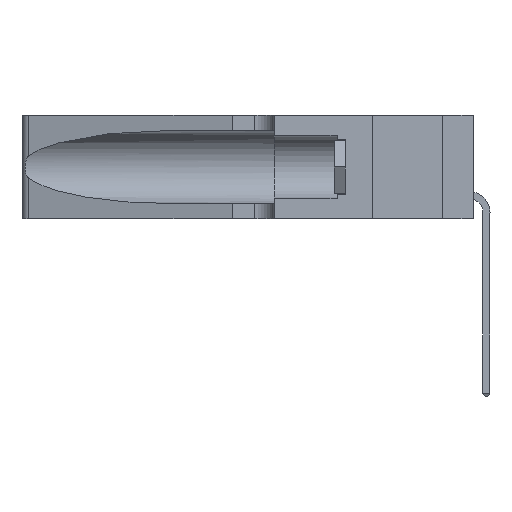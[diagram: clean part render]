
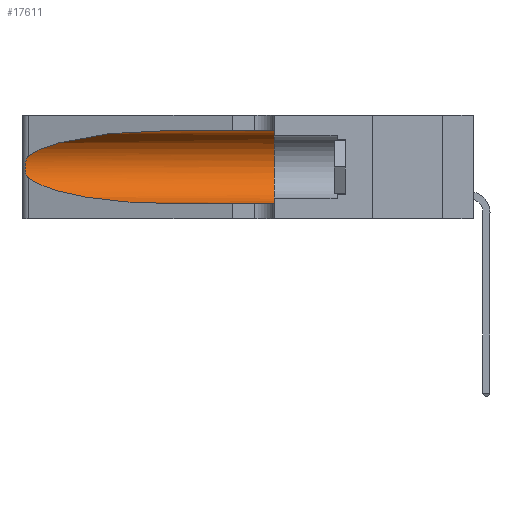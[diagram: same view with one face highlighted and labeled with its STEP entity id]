
A CAD part, left-side view. The second image highlights one B-rep face of the part: STEP entity #17611.
In plain terms, the highlighted cylindrical face has radius 3.308 mm (diameter 6.617 mm), a partial arc.
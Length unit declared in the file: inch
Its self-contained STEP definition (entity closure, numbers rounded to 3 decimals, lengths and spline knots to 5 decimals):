
#126 = VECTOR ( 'NONE', #10944, 39.37008 ) ;
#475 = CARTESIAN_POINT ( 'NONE',  ( 0.25854, 1.2359, 0.20912 ) ) ;
#480 = LINE ( 'NONE', #24969, #126 ) ;
#742 = CARTESIAN_POINT ( 'NONE',  ( 0.25487, 1.22718, 0.14631 ) ) ;
#2258 = CARTESIAN_POINT ( 'NONE',  ( 0.25487, 1.22718, 0.22369 ) ) ;
#2458 = CARTESIAN_POINT ( 'NONE',  ( 0.1305, 0.72297, 0.31525 ) ) ;
#2747 = VERTEX_POINT ( 'NONE', #2458 ) ;
#3385 = CARTESIAN_POINT ( 'NONE',  ( 0.18966, 0.96281, 0.05475 ) ) ;
#4242 = CIRCLE ( 'NONE', #4570, 0.13025 ) ;
#4348 = VERTEX_POINT ( 'NONE', #22023 ) ;
#4570 = AXIS2_PLACEMENT_3D ( 'NONE', #25938, #28212, #21533 ) ;
#4676 = CARTESIAN_POINT ( 'NONE',  ( 0.2373, 1.15595, 0.28018 ) ) ;
#5345 = CYLINDRICAL_SURFACE ( 'NONE', #11756, 0.13025 ) ;
#5872 =( BOUNDED_CURVE ( )  B_SPLINE_CURVE ( 3, ( #13758, #20912, #4676, #2258 ),
 .UNSPECIFIED., .F., .F. ) 
 B_SPLINE_CURVE_WITH_KNOTS ( ( 4, 4 ),
 ( 1.5708, 2.84003 ),
 .UNSPECIFIED. ) 
 CURVE ( )  GEOMETRIC_REPRESENTATION_ITEM ( )  RATIONAL_B_SPLINE_CURVE ( ( 1., 0.87, 0.87, 1. ) ) 
 REPRESENTATION_ITEM ( '' )  );
#6818 = CARTESIAN_POINT ( 'NONE',  ( 0.25487, 1.22718, 0.22369 ) ) ;
#7081 = CARTESIAN_POINT ( 'NONE',  ( 0.25487, 1.22718, 0.22369 ) ) ;
#7170 = CARTESIAN_POINT ( 'NONE',  ( 0.26075, 1.23896, 0.19203 ) ) ;
#7702 = LINE ( 'NONE', #16544, #13161 ) ;
#8995 = FACE_OUTER_BOUND ( 'NONE', #12289, .T. ) ;
#9411 = CARTESIAN_POINT ( 'NONE',  ( 0.25787, 1.23484, 0.2124 ) ) ;
#9726 = CARTESIAN_POINT ( 'NONE',  ( 0.25789, 1.23486, 0.15765 ) ) ;
#9734 = DIRECTION ( 'NONE',  ( 0., -1., 0. ) ) ;
#10086 = CARTESIAN_POINT ( 'NONE',  ( 0.1305, 0.72297, 0.05475 ) ) ;
#10373 = VERTEX_POINT ( 'NONE', #24013 ) ;
#10944 = DIRECTION ( 'NONE',  ( 0., -1., 0. ) ) ;
#11756 = AXIS2_PLACEMENT_3D ( 'NONE', #20277, #27458, #20471 ) ;
#11760 = CARTESIAN_POINT ( 'NONE',  ( 0.25487, 1.22718, 0.14631 ) ) ;
#11892 = ORIENTED_EDGE ( 'NONE', *, *, #30269, .F. ) ;
#12064 = CARTESIAN_POINT ( 'NONE',  ( 0.25555, 1.22993, 0.14849 ) ) ;
#12289 = EDGE_LOOP ( 'NONE', ( #15261, #12811, #27939, #25535, #11892, #27563 ) ) ;
#12811 = ORIENTED_EDGE ( 'NONE', *, *, #29656, .T. ) ;
#12876 = EDGE_CURVE ( 'NONE', #2747, #17040, #7702, .T. ) ;
#13161 = VECTOR ( 'NONE', #9734, 39.37008 ) ;
#13758 = CARTESIAN_POINT ( 'NONE',  ( 0.1305, 0.72297, 0.31525 ) ) ;
#15035 = CARTESIAN_POINT ( 'NONE',  ( 0.1305, 0.35, 0.31525 ) ) ;
#15261 = ORIENTED_EDGE ( 'NONE', *, *, #25321, .T. ) ;
#15842 = VERTEX_POINT ( 'NONE', #6818 ) ;
#16496 =( BOUNDED_CURVE ( )  B_SPLINE_CURVE ( 3, ( #742, #17305, #3385, #10086 ),
 .UNSPECIFIED., .F., .F. ) 
 B_SPLINE_CURVE_WITH_KNOTS ( ( 4, 4 ),
 ( 3.44316, 4.71239 ),
 .UNSPECIFIED. ) 
 CURVE ( )  GEOMETRIC_REPRESENTATION_ITEM ( )  RATIONAL_B_SPLINE_CURVE ( ( 1., 0.87, 0.87, 1. ) ) 
 REPRESENTATION_ITEM ( '' )  );
#16544 = CARTESIAN_POINT ( 'NONE',  ( 0.1305, 1.61858, 0.31525 ) ) ;
#17040 = VERTEX_POINT ( 'NONE', #15035 ) ;
#17305 = CARTESIAN_POINT ( 'NONE',  ( 0.2373, 1.15595, 0.08982 ) ) ;
#17611 = ADVANCED_FACE ( 'NONE', ( #8995 ), #5345, .F. ) ;
#19512 = B_SPLINE_CURVE_WITH_KNOTS ( 'NONE', 3,
 ( #7081, #25869, #28455, #9411, #475, #28153, #7170, #21375, #25780, #23752, #9726, #23541, #12064, #11760 ),
 .UNSPECIFIED., .F., .F.,
 ( 4, 2, 2, 2, 2, 2, 4 ),
 ( 0., 0.00027, 0.00053, 0.00107, 0.0016, 0.00187, 0.00214 ),
 .UNSPECIFIED. ) ;
#20108 = EDGE_CURVE ( 'NONE', #10373, #22049, #480, .T. ) ;
#20277 = CARTESIAN_POINT ( 'NONE',  ( 0.1305, 1.61858, 0.185 ) ) ;
#20471 = DIRECTION ( 'NONE',  ( 0., 0., -1. ) ) ;
#20912 = CARTESIAN_POINT ( 'NONE',  ( 0.18966, 0.96281, 0.31525 ) ) ;
#21375 = CARTESIAN_POINT ( 'NONE',  ( 0.26075, 1.23896, 0.178 ) ) ;
#21533 = DIRECTION ( 'NONE',  ( 0., 0., 1. ) ) ;
#22023 = CARTESIAN_POINT ( 'NONE',  ( 0.25487, 1.22718, 0.14631 ) ) ;
#22049 = VERTEX_POINT ( 'NONE', #22128 ) ;
#22128 = CARTESIAN_POINT ( 'NONE',  ( 0.1305, 0.35, 0.05475 ) ) ;
#23541 = CARTESIAN_POINT ( 'NONE',  ( 0.25639, 1.23186, 0.15144 ) ) ;
#23719 = EDGE_CURVE ( 'NONE', #4348, #10373, #16496, .T. ) ;
#23752 = CARTESIAN_POINT ( 'NONE',  ( 0.25856, 1.23593, 0.16098 ) ) ;
#24013 = CARTESIAN_POINT ( 'NONE',  ( 0.1305, 0.72297, 0.05475 ) ) ;
#24969 = CARTESIAN_POINT ( 'NONE',  ( 0.1305, 1.61858, 0.05475 ) ) ;
#25321 = EDGE_CURVE ( 'NONE', #2747, #15842, #5872, .T. ) ;
#25535 = ORIENTED_EDGE ( 'NONE', *, *, #20108, .T. ) ;
#25780 = CARTESIAN_POINT ( 'NONE',  ( 0.26017, 1.23833, 0.17102 ) ) ;
#25869 = CARTESIAN_POINT ( 'NONE',  ( 0.25555, 1.22994, 0.2215 ) ) ;
#25938 = CARTESIAN_POINT ( 'NONE',  ( 0.1305, 0.35, 0.185 ) ) ;
#27458 = DIRECTION ( 'NONE',  ( 0., -1., 0. ) ) ;
#27563 = ORIENTED_EDGE ( 'NONE', *, *, #12876, .F. ) ;
#27939 = ORIENTED_EDGE ( 'NONE', *, *, #23719, .T. ) ;
#28153 = CARTESIAN_POINT ( 'NONE',  ( 0.26018, 1.23835, 0.19895 ) ) ;
#28212 = DIRECTION ( 'NONE',  ( 0., 1., 0. ) ) ;
#28455 = CARTESIAN_POINT ( 'NONE',  ( 0.25639, 1.23184, 0.21858 ) ) ;
#29656 = EDGE_CURVE ( 'NONE', #15842, #4348, #19512, .T. ) ;
#30269 = EDGE_CURVE ( 'NONE', #17040, #22049, #4242, .T. ) ;
